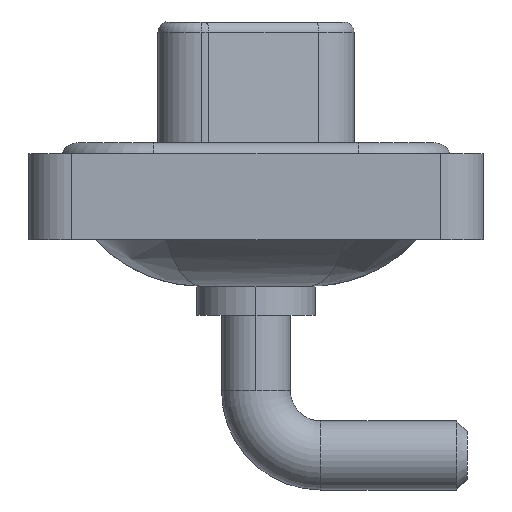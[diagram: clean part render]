
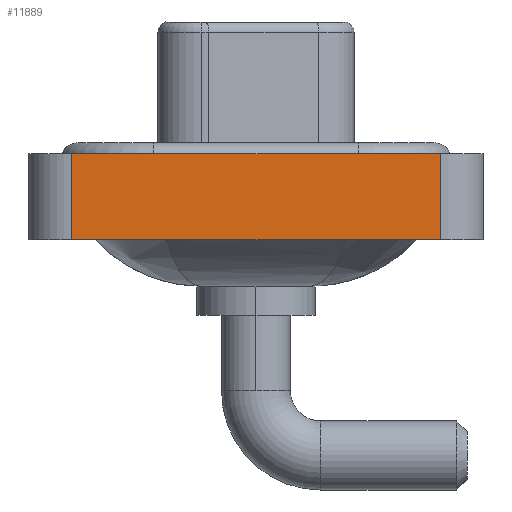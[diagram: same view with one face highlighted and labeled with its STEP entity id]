
A CAD part, left-side view. The second image highlights one B-rep face of the part: STEP entity #11889.
In plain terms, the highlighted planar face has unit normal (-1, 0, 0).
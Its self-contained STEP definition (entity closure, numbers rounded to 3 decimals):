
#75 = VECTOR ( 'NONE', #4711, 1000. ) ;
#736 = CARTESIAN_POINT ( 'NONE',  ( -7.3, -8.55, 0.4 ) ) ;
#994 = CARTESIAN_POINT ( 'NONE',  ( -7.3, 8.55, -3.6 ) ) ;
#1109 = EDGE_CURVE ( 'NONE', #13246, #3745, #7060, .T. ) ;
#1194 = AXIS2_PLACEMENT_3D ( 'NONE', #4734, #9931, #9843 ) ;
#1298 = CARTESIAN_POINT ( 'NONE',  ( -7.3, -8.55, -3.6 ) ) ;
#2359 = EDGE_LOOP ( 'NONE', ( #4840, #11263, #10494, #14129 ) ) ;
#3021 = VECTOR ( 'NONE', #12201, 1000. ) ;
#3745 = VERTEX_POINT ( 'NONE', #6605 ) ;
#3959 = LINE ( 'NONE', #1298, #14855 ) ;
#4711 = DIRECTION ( 'NONE',  ( 0., 0., 1. ) ) ;
#4734 = CARTESIAN_POINT ( 'NONE',  ( -7.3, -8.55, -3.6 ) ) ;
#4840 = ORIENTED_EDGE ( 'NONE', *, *, #13183, .T. ) ;
#5843 = EDGE_CURVE ( 'NONE', #11877, #13246, #8475, .T. ) ;
#5846 = CARTESIAN_POINT ( 'NONE',  ( -7.3, -8.55, -3.6 ) ) ;
#6015 = CARTESIAN_POINT ( 'NONE',  ( -7.3, 8.55, 0.4 ) ) ;
#6605 = CARTESIAN_POINT ( 'NONE',  ( -7.3, -8.55, 0.4 ) ) ;
#7060 = LINE ( 'NONE', #736, #3021 ) ;
#8371 = LINE ( 'NONE', #5846, #16450 ) ;
#8475 = LINE ( 'NONE', #14849, #75 ) ;
#8528 = DIRECTION ( 'NONE',  ( 0., 0., 1. ) ) ;
#9843 = DIRECTION ( 'NONE',  ( 0., 0., 1. ) ) ;
#9931 = DIRECTION ( 'NONE',  ( -1., 0., 0. ) ) ;
#10494 = ORIENTED_EDGE ( 'NONE', *, *, #5843, .F. ) ;
#11263 = ORIENTED_EDGE ( 'NONE', *, *, #1109, .F. ) ;
#11877 = VERTEX_POINT ( 'NONE', #994 ) ;
#11889 = ADVANCED_FACE ( 'NONE', ( #12463 ), #16285, .T. ) ;
#12201 = DIRECTION ( 'NONE',  ( 0., -1., 0. ) ) ;
#12463 = FACE_OUTER_BOUND ( 'NONE', #2359, .T. ) ;
#12571 = VERTEX_POINT ( 'NONE', #16518 ) ;
#12983 = EDGE_CURVE ( 'NONE', #11877, #12571, #3959, .T. ) ;
#13183 = EDGE_CURVE ( 'NONE', #12571, #3745, #8371, .T. ) ;
#13246 = VERTEX_POINT ( 'NONE', #6015 ) ;
#14089 = DIRECTION ( 'NONE',  ( 0., -1., 0. ) ) ;
#14129 = ORIENTED_EDGE ( 'NONE', *, *, #12983, .T. ) ;
#14849 = CARTESIAN_POINT ( 'NONE',  ( -7.3, 8.55, -3.6 ) ) ;
#14855 = VECTOR ( 'NONE', #14089, 1000. ) ;
#16285 = PLANE ( 'NONE',  #1194 ) ;
#16450 = VECTOR ( 'NONE', #8528, 1000. ) ;
#16518 = CARTESIAN_POINT ( 'NONE',  ( -7.3, -8.55, -3.6 ) ) ;
